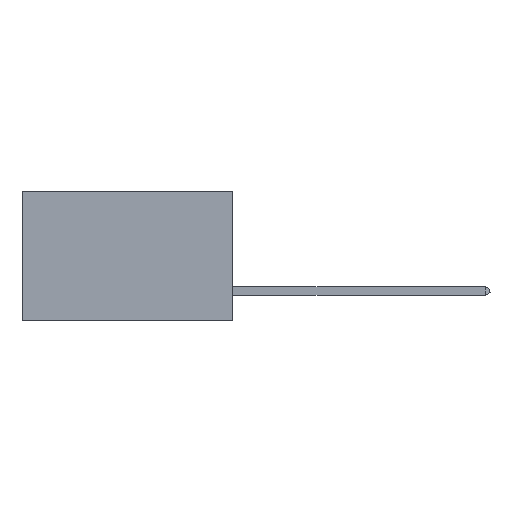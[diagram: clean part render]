
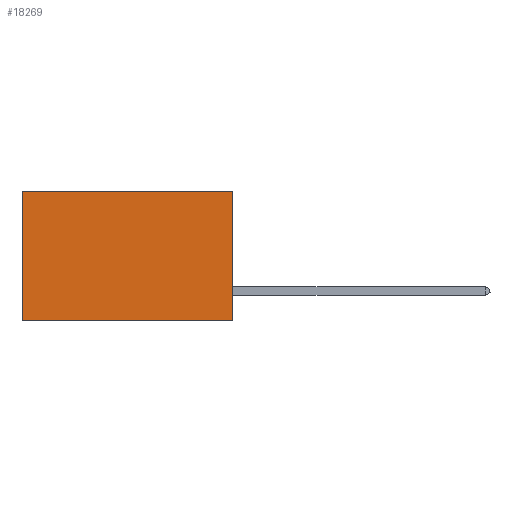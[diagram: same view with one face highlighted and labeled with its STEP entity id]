
A CAD part, left-side view. The second image highlights one B-rep face of the part: STEP entity #18269.
In plain terms, the highlighted planar face has unit normal (-1, 0, 0).
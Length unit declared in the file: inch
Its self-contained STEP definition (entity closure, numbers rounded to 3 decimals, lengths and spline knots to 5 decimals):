
#1043 = DIRECTION ( 'NONE',  ( 0., 1., 0. ) ) ;
#1966 = ORIENTED_EDGE ( 'NONE', *, *, #25609, .F. ) ;
#1986 = CARTESIAN_POINT ( 'NONE',  ( 0.2875, 0., 0. ) ) ;
#1988 = LINE ( 'NONE', #14330, #29196 ) ;
#2198 = DIRECTION ( 'NONE',  ( 0., 0., -1. ) ) ;
#4011 = VECTOR ( 'NONE', #9829, 39.37008 ) ;
#6574 = CARTESIAN_POINT ( 'NONE',  ( 0.2875, 0.6, 0. ) ) ;
#7235 = VECTOR ( 'NONE', #1043, 39.37008 ) ;
#8535 = CARTESIAN_POINT ( 'NONE',  ( 0.2875, 0., -0.37 ) ) ;
#9746 = VERTEX_POINT ( 'NONE', #18216 ) ;
#9829 = DIRECTION ( 'NONE',  ( 0., 0., -1. ) ) ;
#10295 = EDGE_LOOP ( 'NONE', ( #23612, #16497, #1966, #17456 ) ) ;
#10842 = LINE ( 'NONE', #21600, #4011 ) ;
#11799 = EDGE_CURVE ( 'NONE', #9746, #30736, #1988, .T. ) ;
#11802 = DIRECTION ( 'NONE',  ( 0., 1., 0. ) ) ;
#11884 = AXIS2_PLACEMENT_3D ( 'NONE', #1986, #30845, #21378 ) ;
#11885 = CARTESIAN_POINT ( 'NONE',  ( 0.2875, 0.6, -0.37 ) ) ;
#11886 = VERTEX_POINT ( 'NONE', #11885 ) ;
#14330 = CARTESIAN_POINT ( 'NONE',  ( 0.2875, 0., 0. ) ) ;
#14563 = EDGE_CURVE ( 'NONE', #23082, #11886, #15939, .T. ) ;
#15939 = LINE ( 'NONE', #22763, #7235 ) ;
#16497 = ORIENTED_EDGE ( 'NONE', *, *, #14563, .F. ) ;
#16539 = LINE ( 'NONE', #26458, #29355 ) ;
#17456 = ORIENTED_EDGE ( 'NONE', *, *, #11799, .T. ) ;
#18216 = CARTESIAN_POINT ( 'NONE',  ( 0.2875, 0., 0. ) ) ;
#18269 = ADVANCED_FACE ( 'NONE', ( #30033 ), #18973, .F. ) ;
#18973 = PLANE ( 'NONE',  #11884 ) ;
#21378 = DIRECTION ( 'NONE',  ( 0., 0., -1. ) ) ;
#21600 = CARTESIAN_POINT ( 'NONE',  ( 0.2875, 0.6, 0. ) ) ;
#22763 = CARTESIAN_POINT ( 'NONE',  ( 0.2875, 0., -0.37 ) ) ;
#23082 = VERTEX_POINT ( 'NONE', #8535 ) ;
#23612 = ORIENTED_EDGE ( 'NONE', *, *, #29614, .T. ) ;
#25609 = EDGE_CURVE ( 'NONE', #9746, #23082, #16539, .T. ) ;
#26458 = CARTESIAN_POINT ( 'NONE',  ( 0.2875, 0., 0. ) ) ;
#29196 = VECTOR ( 'NONE', #11802, 39.37008 ) ;
#29355 = VECTOR ( 'NONE', #2198, 39.37008 ) ;
#29614 = EDGE_CURVE ( 'NONE', #30736, #11886, #10842, .T. ) ;
#30033 = FACE_OUTER_BOUND ( 'NONE', #10295, .T. ) ;
#30736 = VERTEX_POINT ( 'NONE', #6574 ) ;
#30845 = DIRECTION ( 'NONE',  ( 1., 0., 0. ) ) ;
